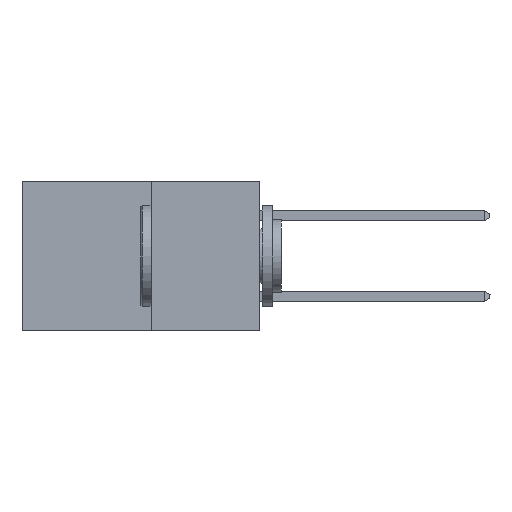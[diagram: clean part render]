
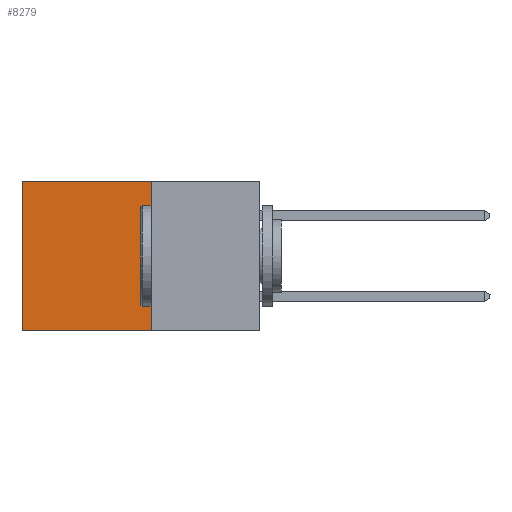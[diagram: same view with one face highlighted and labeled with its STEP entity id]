
A CAD part, left-side view. The second image highlights one B-rep face of the part: STEP entity #8279.
In plain terms, the highlighted planar face has unit normal (-1, 0, 0).
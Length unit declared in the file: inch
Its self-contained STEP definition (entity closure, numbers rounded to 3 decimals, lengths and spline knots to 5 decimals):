
#450 = LINE ( 'NONE', #5384, #22106 ) ;
#1350 = ORIENTED_EDGE ( 'NONE', *, *, #21499, .T. ) ;
#2257 = VERTEX_POINT ( 'NONE', #26386 ) ;
#3240 = VERTEX_POINT ( 'NONE', #20008 ) ;
#3673 = LINE ( 'NONE', #7077, #14817 ) ;
#5384 = CARTESIAN_POINT ( 'NONE',  ( 0.277, 0.59, -0.37 ) ) ;
#5686 = VERTEX_POINT ( 'NONE', #25271 ) ;
#6604 = EDGE_CURVE ( 'NONE', #2257, #3240, #13428, .T. ) ;
#6730 = CARTESIAN_POINT ( 'NONE',  ( 0.277, 0.59, 0. ) ) ;
#7077 = CARTESIAN_POINT ( 'NONE',  ( 0.277, 0.27, -0.37 ) ) ;
#7531 = DIRECTION ( 'NONE',  ( 0., 0., -1. ) ) ;
#7545 = VECTOR ( 'NONE', #22585, 39.37008 ) ;
#8279 = ADVANCED_FACE ( 'NONE', ( #17273 ), #10827, .F. ) ;
#9880 = VERTEX_POINT ( 'NONE', #6730 ) ;
#10057 = CARTESIAN_POINT ( 'NONE',  ( 0.277, 0.27, 0. ) ) ;
#10663 = DIRECTION ( 'NONE',  ( 0., 0., -1. ) ) ;
#10796 = DIRECTION ( 'NONE',  ( 1., 0., 0. ) ) ;
#10827 = PLANE ( 'NONE',  #24966 ) ;
#11744 = CARTESIAN_POINT ( 'NONE',  ( 0.277, 0.27, -0.37 ) ) ;
#12058 = ORIENTED_EDGE ( 'NONE', *, *, #19128, .F. ) ;
#12766 = ORIENTED_EDGE ( 'NONE', *, *, #17452, .T. ) ;
#13093 = LINE ( 'NONE', #10057, #7545 ) ;
#13428 = LINE ( 'NONE', #14624, #18332 ) ;
#13556 = EDGE_LOOP ( 'NONE', ( #12766, #16108, #12058, #1350 ) ) ;
#14526 = DIRECTION ( 'NONE',  ( 0., 1., 0. ) ) ;
#14624 = CARTESIAN_POINT ( 'NONE',  ( 0.277, 0.27, -0.37 ) ) ;
#14817 = VECTOR ( 'NONE', #21708, 39.37008 ) ;
#16108 = ORIENTED_EDGE ( 'NONE', *, *, #6604, .F. ) ;
#17273 = FACE_OUTER_BOUND ( 'NONE', #13556, .T. ) ;
#17452 = EDGE_CURVE ( 'NONE', #9880, #3240, #450, .T. ) ;
#18332 = VECTOR ( 'NONE', #14526, 39.37008 ) ;
#19128 = EDGE_CURVE ( 'NONE', #5686, #2257, #3673, .T. ) ;
#20008 = CARTESIAN_POINT ( 'NONE',  ( 0.277, 0.59, -0.37 ) ) ;
#21499 = EDGE_CURVE ( 'NONE', #5686, #9880, #13093, .T. ) ;
#21708 = DIRECTION ( 'NONE',  ( 0., 0., -1. ) ) ;
#22106 = VECTOR ( 'NONE', #7531, 39.37008 ) ;
#22585 = DIRECTION ( 'NONE',  ( 0., 1., 0. ) ) ;
#24966 = AXIS2_PLACEMENT_3D ( 'NONE', #11744, #10796, #10663 ) ;
#25271 = CARTESIAN_POINT ( 'NONE',  ( 0.277, 0.27, 0. ) ) ;
#26386 = CARTESIAN_POINT ( 'NONE',  ( 0.277, 0.27, -0.37 ) ) ;
